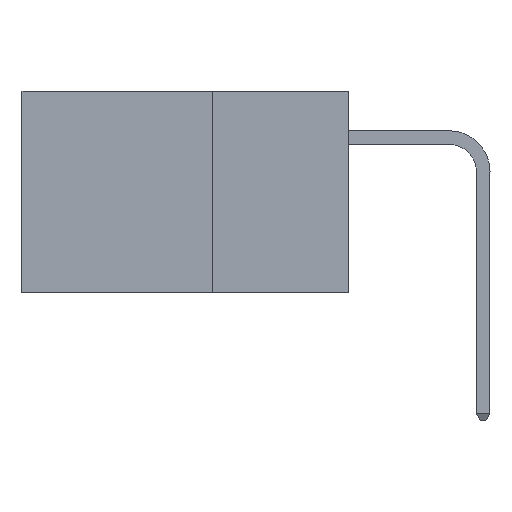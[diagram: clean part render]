
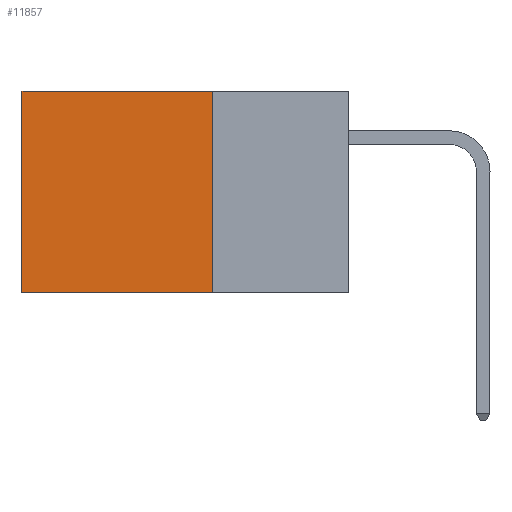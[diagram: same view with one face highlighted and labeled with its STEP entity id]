
A CAD part, left-side view. The second image highlights one B-rep face of the part: STEP entity #11857.
In plain terms, the highlighted planar face has unit normal (-1, 0, 0).
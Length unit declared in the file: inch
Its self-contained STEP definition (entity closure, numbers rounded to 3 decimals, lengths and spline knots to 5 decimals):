
#665 = DIRECTION ( 'NONE',  ( 0., 0., -1. ) ) ;
#1488 = VERTEX_POINT ( 'NONE', #11838 ) ;
#1524 = EDGE_LOOP ( 'NONE', ( #8344, #15196, #6894, #4257 ) ) ;
#1957 = CARTESIAN_POINT ( 'NONE',  ( 0.2875, 0.6, -0.37 ) ) ;
#2056 = CARTESIAN_POINT ( 'NONE',  ( 0.2875, 0.25, 0. ) ) ;
#2202 = LINE ( 'NONE', #2056, #3571 ) ;
#2947 = EDGE_CURVE ( 'NONE', #11221, #1488, #2202, .T. ) ;
#3093 = EDGE_CURVE ( 'NONE', #11221, #12665, #7618, .T. ) ;
#3178 = DIRECTION ( 'NONE',  ( 0., 0., -1. ) ) ;
#3571 = VECTOR ( 'NONE', #7098, 39.37008 ) ;
#3783 = VECTOR ( 'NONE', #665, 39.37008 ) ;
#4257 = ORIENTED_EDGE ( 'NONE', *, *, #2947, .T. ) ;
#4366 = CARTESIAN_POINT ( 'NONE',  ( 0.2875, 0.25, 0. ) ) ;
#4411 = CARTESIAN_POINT ( 'NONE',  ( 0.2875, 0.25, -0.37 ) ) ;
#5695 = DIRECTION ( 'NONE',  ( 1., 0., 0. ) ) ;
#5839 = CARTESIAN_POINT ( 'NONE',  ( 0.2875, 0.25, -0.37 ) ) ;
#5892 = PLANE ( 'NONE',  #7779 ) ;
#6894 = ORIENTED_EDGE ( 'NONE', *, *, #3093, .F. ) ;
#7098 = DIRECTION ( 'NONE',  ( 0., 1., 0. ) ) ;
#7544 = EDGE_CURVE ( 'NONE', #12665, #9819, #10361, .T. ) ;
#7618 = LINE ( 'NONE', #12067, #3783 ) ;
#7779 = AXIS2_PLACEMENT_3D ( 'NONE', #4366, #5695, #15957 ) ;
#8344 = ORIENTED_EDGE ( 'NONE', *, *, #9188, .T. ) ;
#8588 = CARTESIAN_POINT ( 'NONE',  ( 0.2875, 0.25, 0. ) ) ;
#9188 = EDGE_CURVE ( 'NONE', #1488, #9819, #15601, .T. ) ;
#9819 = VERTEX_POINT ( 'NONE', #1957 ) ;
#10361 = LINE ( 'NONE', #5839, #14003 ) ;
#10552 = FACE_OUTER_BOUND ( 'NONE', #1524, .T. ) ;
#11221 = VERTEX_POINT ( 'NONE', #8588 ) ;
#11838 = CARTESIAN_POINT ( 'NONE',  ( 0.2875, 0.6, 0. ) ) ;
#11857 = ADVANCED_FACE ( 'NONE', ( #10552 ), #5892, .F. ) ;
#12067 = CARTESIAN_POINT ( 'NONE',  ( 0.2875, 0.25, 0. ) ) ;
#12665 = VERTEX_POINT ( 'NONE', #4411 ) ;
#13138 = VECTOR ( 'NONE', #3178, 39.37008 ) ;
#14003 = VECTOR ( 'NONE', #18619, 39.37008 ) ;
#15196 = ORIENTED_EDGE ( 'NONE', *, *, #7544, .F. ) ;
#15601 = LINE ( 'NONE', #17671, #13138 ) ;
#15957 = DIRECTION ( 'NONE',  ( 0., 0., -1. ) ) ;
#17671 = CARTESIAN_POINT ( 'NONE',  ( 0.2875, 0.6, 0. ) ) ;
#18619 = DIRECTION ( 'NONE',  ( 0., 1., 0. ) ) ;
